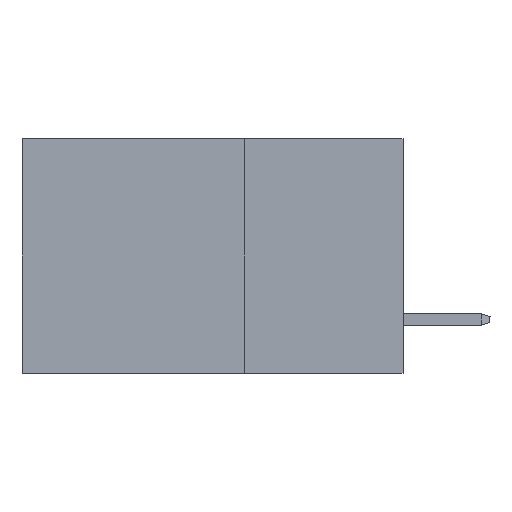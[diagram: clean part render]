
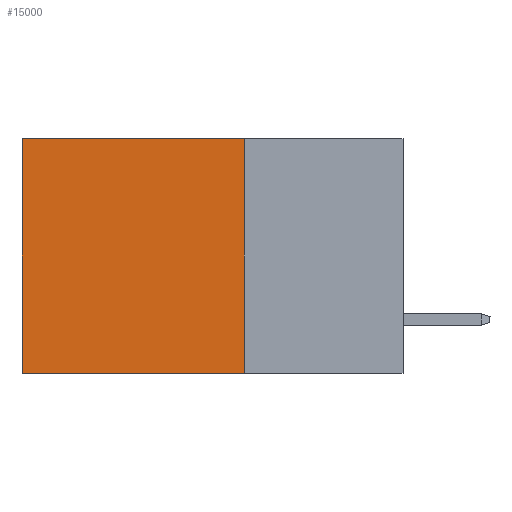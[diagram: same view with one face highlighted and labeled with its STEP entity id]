
A CAD part, left-side view. The second image highlights one B-rep face of the part: STEP entity #15000.
In plain terms, the highlighted planar face has unit normal (-1, 0, 0).
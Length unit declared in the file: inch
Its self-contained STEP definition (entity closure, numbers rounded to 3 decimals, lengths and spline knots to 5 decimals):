
#957 = ORIENTED_EDGE ( 'NONE', *, *, #19967, .F. ) ;
#1278 = CARTESIAN_POINT ( 'NONE',  ( 0.2875, 0.25, 0. ) ) ;
#5840 = DIRECTION ( 'NONE',  ( 0., 0., -1. ) ) ;
#6283 = EDGE_CURVE ( 'NONE', #9626, #10153, #18353, .T. ) ;
#7078 = LINE ( 'NONE', #15353, #15227 ) ;
#7942 = ORIENTED_EDGE ( 'NONE', *, *, #17966, .T. ) ;
#8641 = DIRECTION ( 'NONE',  ( 0., 1., 0. ) ) ;
#9626 = VERTEX_POINT ( 'NONE', #14802 ) ;
#10087 = CARTESIAN_POINT ( 'NONE',  ( 0.2875, 0.25, -0.37 ) ) ;
#10153 = VERTEX_POINT ( 'NONE', #10087 ) ;
#10718 = PLANE ( 'NONE',  #19061 ) ;
#12010 = EDGE_CURVE ( 'NONE', #14463, #14993, #14726, .T. ) ;
#12148 = VECTOR ( 'NONE', #18804, 39.37008 ) ;
#12481 = CARTESIAN_POINT ( 'NONE',  ( 0.2875, 0.6, -0.37 ) ) ;
#12923 = CARTESIAN_POINT ( 'NONE',  ( 0.2875, 0.6, 0. ) ) ;
#13656 = ORIENTED_EDGE ( 'NONE', *, *, #6283, .F. ) ;
#14360 = VECTOR ( 'NONE', #19671, 39.37008 ) ;
#14463 = VERTEX_POINT ( 'NONE', #12923 ) ;
#14726 = LINE ( 'NONE', #21442, #15869 ) ;
#14802 = CARTESIAN_POINT ( 'NONE',  ( 0.2875, 0.25, 0. ) ) ;
#14993 = VERTEX_POINT ( 'NONE', #12481 ) ;
#15000 = ADVANCED_FACE ( 'NONE', ( #16195 ), #10718, .F. ) ;
#15227 = VECTOR ( 'NONE', #8641, 39.37008 ) ;
#15353 = CARTESIAN_POINT ( 'NONE',  ( 0.2875, 0.25, -0.37 ) ) ;
#15507 = EDGE_LOOP ( 'NONE', ( #18442, #957, #13656, #7942 ) ) ;
#15869 = VECTOR ( 'NONE', #16054, 39.37008 ) ;
#16054 = DIRECTION ( 'NONE',  ( 0., 0., -1. ) ) ;
#16195 = FACE_OUTER_BOUND ( 'NONE', #15507, .T. ) ;
#16927 = CARTESIAN_POINT ( 'NONE',  ( 0.2875, 0.25, 0. ) ) ;
#17145 = LINE ( 'NONE', #16927, #12148 ) ;
#17425 = CARTESIAN_POINT ( 'NONE',  ( 0.2875, 0.25, 0. ) ) ;
#17760 = DIRECTION ( 'NONE',  ( 1., 0., 0. ) ) ;
#17966 = EDGE_CURVE ( 'NONE', #9626, #14463, #17145, .T. ) ;
#18353 = LINE ( 'NONE', #1278, #14360 ) ;
#18442 = ORIENTED_EDGE ( 'NONE', *, *, #12010, .T. ) ;
#18804 = DIRECTION ( 'NONE',  ( 0., 1., 0. ) ) ;
#19061 = AXIS2_PLACEMENT_3D ( 'NONE', #17425, #17760, #5840 ) ;
#19671 = DIRECTION ( 'NONE',  ( 0., 0., -1. ) ) ;
#19967 = EDGE_CURVE ( 'NONE', #10153, #14993, #7078, .T. ) ;
#21442 = CARTESIAN_POINT ( 'NONE',  ( 0.2875, 0.6, 0. ) ) ;
